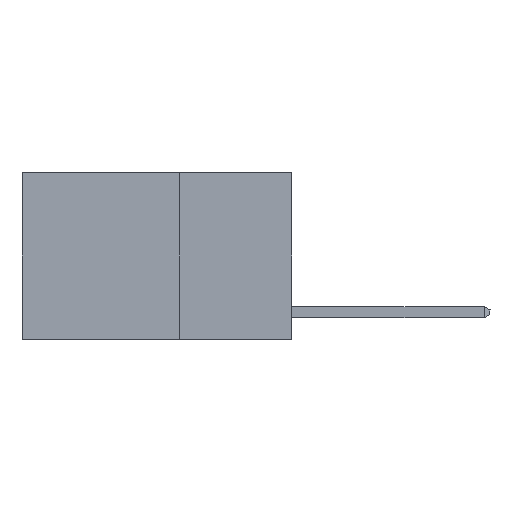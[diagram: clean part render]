
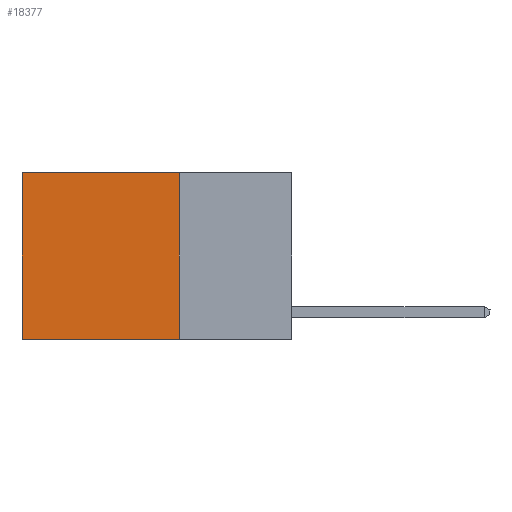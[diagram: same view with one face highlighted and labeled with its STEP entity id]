
A CAD part, left-side view. The second image highlights one B-rep face of the part: STEP entity #18377.
In plain terms, the highlighted planar face has unit normal (-1, 0, 0).
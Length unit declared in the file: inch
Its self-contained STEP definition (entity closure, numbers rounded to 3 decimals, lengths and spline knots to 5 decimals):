
#68 = VECTOR ( 'NONE', #19820, 39.37008 ) ;
#572 = DIRECTION ( 'NONE',  ( 0., 0., -1. ) ) ;
#3211 = CARTESIAN_POINT ( 'NONE',  ( 0.2625, 0.25, 0. ) ) ;
#4601 = DIRECTION ( 'NONE',  ( 0., 1., 0. ) ) ;
#4693 = VERTEX_POINT ( 'NONE', #25098 ) ;
#5643 = VERTEX_POINT ( 'NONE', #19897 ) ;
#6195 = EDGE_LOOP ( 'NONE', ( #28464, #19236, #24148, #16494 ) ) ;
#6320 = EDGE_CURVE ( 'NONE', #4693, #26573, #19188, .T. ) ;
#6407 = EDGE_CURVE ( 'NONE', #14534, #26573, #11139, .T. ) ;
#10062 = DIRECTION ( 'NONE',  ( 1., 0., 0. ) ) ;
#10443 = VECTOR ( 'NONE', #22834, 39.37008 ) ;
#10706 = VECTOR ( 'NONE', #572, 39.37008 ) ;
#10845 = CARTESIAN_POINT ( 'NONE',  ( 0.2625, 0.25, 0. ) ) ;
#11139 = LINE ( 'NONE', #27296, #10443 ) ;
#12089 = LINE ( 'NONE', #10845, #68 ) ;
#13390 = FACE_OUTER_BOUND ( 'NONE', #6195, .T. ) ;
#14534 = VERTEX_POINT ( 'NONE', #24079 ) ;
#16217 = EDGE_CURVE ( 'NONE', #5643, #14534, #12089, .T. ) ;
#16350 = CARTESIAN_POINT ( 'NONE',  ( 0.2625, 0.25, 0. ) ) ;
#16494 = ORIENTED_EDGE ( 'NONE', *, *, #16217, .T. ) ;
#17359 = LINE ( 'NONE', #16350, #10706 ) ;
#18377 = ADVANCED_FACE ( 'NONE', ( #13390 ), #23418, .F. ) ;
#19188 = LINE ( 'NONE', #20335, #24383 ) ;
#19236 = ORIENTED_EDGE ( 'NONE', *, *, #6320, .F. ) ;
#19820 = DIRECTION ( 'NONE',  ( 0., 1., 0. ) ) ;
#19897 = CARTESIAN_POINT ( 'NONE',  ( 0.2625, 0.25, 0. ) ) ;
#20335 = CARTESIAN_POINT ( 'NONE',  ( 0.2625, 0.25, -0.37 ) ) ;
#22688 = AXIS2_PLACEMENT_3D ( 'NONE', #3211, #10062, #25633 ) ;
#22834 = DIRECTION ( 'NONE',  ( 0., 0., -1. ) ) ;
#23418 = PLANE ( 'NONE',  #22688 ) ;
#24079 = CARTESIAN_POINT ( 'NONE',  ( 0.2625, 0.6, 0. ) ) ;
#24148 = ORIENTED_EDGE ( 'NONE', *, *, #27024, .F. ) ;
#24383 = VECTOR ( 'NONE', #4601, 39.37008 ) ;
#25098 = CARTESIAN_POINT ( 'NONE',  ( 0.2625, 0.25, -0.37 ) ) ;
#25633 = DIRECTION ( 'NONE',  ( 0., 0., -1. ) ) ;
#25980 = CARTESIAN_POINT ( 'NONE',  ( 0.2625, 0.6, -0.37 ) ) ;
#26573 = VERTEX_POINT ( 'NONE', #25980 ) ;
#27024 = EDGE_CURVE ( 'NONE', #5643, #4693, #17359, .T. ) ;
#27296 = CARTESIAN_POINT ( 'NONE',  ( 0.2625, 0.6, 0. ) ) ;
#28464 = ORIENTED_EDGE ( 'NONE', *, *, #6407, .T. ) ;
